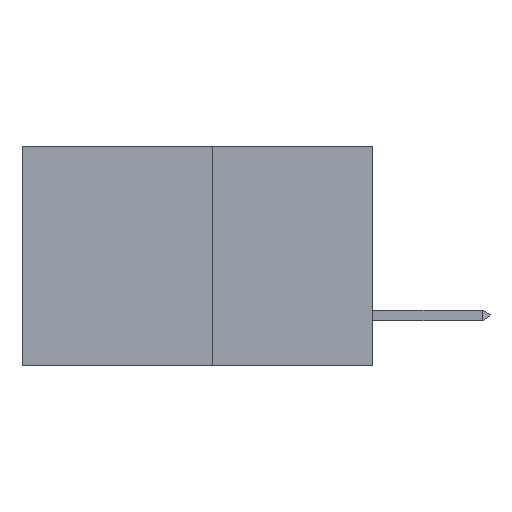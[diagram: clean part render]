
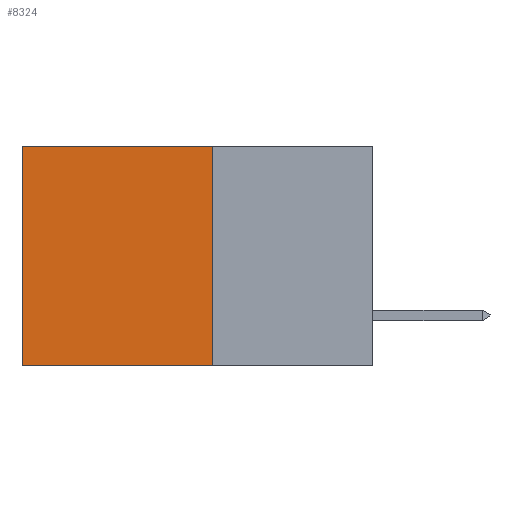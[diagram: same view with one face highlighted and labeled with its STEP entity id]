
A CAD part, left-side view. The second image highlights one B-rep face of the part: STEP entity #8324.
In plain terms, the highlighted planar face has unit normal (-1, 0, 0).
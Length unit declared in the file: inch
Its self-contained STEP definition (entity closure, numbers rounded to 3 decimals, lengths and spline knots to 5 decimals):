
#321 = VECTOR ( 'NONE', #8732, 39.37008 ) ;
#1023 = EDGE_CURVE ( 'NONE', #16219, #23307, #23272, .T. ) ;
#2029 = ORIENTED_EDGE ( 'NONE', *, *, #27375, .T. ) ;
#3308 = CARTESIAN_POINT ( 'NONE',  ( 0.277, 0.27, 0. ) ) ;
#4732 = LINE ( 'NONE', #7775, #20973 ) ;
#4986 = PLANE ( 'NONE',  #8059 ) ;
#6229 = EDGE_CURVE ( 'NONE', #21090, #7030, #11369, .T. ) ;
#7030 = VERTEX_POINT ( 'NONE', #16469 ) ;
#7775 = CARTESIAN_POINT ( 'NONE',  ( 0.277, 0.27, 0. ) ) ;
#8059 = AXIS2_PLACEMENT_3D ( 'NONE', #22584, #9438, #24719 ) ;
#8324 = ADVANCED_FACE ( 'NONE', ( #8785 ), #4986, .F. ) ;
#8732 = DIRECTION ( 'NONE',  ( 0., 0., -1. ) ) ;
#8767 = CARTESIAN_POINT ( 'NONE',  ( 0.277, 0.27, -0.37 ) ) ;
#8777 = ORIENTED_EDGE ( 'NONE', *, *, #9571, .F. ) ;
#8785 = FACE_OUTER_BOUND ( 'NONE', #26410, .T. ) ;
#9438 = DIRECTION ( 'NONE',  ( 1., 0., 0. ) ) ;
#9571 = EDGE_CURVE ( 'NONE', #7030, #23307, #25844, .T. ) ;
#9575 = DIRECTION ( 'NONE',  ( 0., 1., 0. ) ) ;
#11369 = LINE ( 'NONE', #8767, #321 ) ;
#13594 = ORIENTED_EDGE ( 'NONE', *, *, #6229, .F. ) ;
#14039 = DIRECTION ( 'NONE',  ( 0., 0., -1. ) ) ;
#14264 = CARTESIAN_POINT ( 'NONE',  ( 0.277, 0.59, -0.37 ) ) ;
#14354 = VECTOR ( 'NONE', #9575, 39.37008 ) ;
#15816 = CARTESIAN_POINT ( 'NONE',  ( 0.277, 0.59, -0.37 ) ) ;
#16219 = VERTEX_POINT ( 'NONE', #21399 ) ;
#16469 = CARTESIAN_POINT ( 'NONE',  ( 0.277, 0.27, -0.37 ) ) ;
#20973 = VECTOR ( 'NONE', #20998, 39.37008 ) ;
#20998 = DIRECTION ( 'NONE',  ( 0., 1., 0. ) ) ;
#21090 = VERTEX_POINT ( 'NONE', #3308 ) ;
#21399 = CARTESIAN_POINT ( 'NONE',  ( 0.277, 0.59, 0. ) ) ;
#22584 = CARTESIAN_POINT ( 'NONE',  ( 0.277, 0.27, -0.37 ) ) ;
#22601 = VECTOR ( 'NONE', #14039, 39.37008 ) ;
#23272 = LINE ( 'NONE', #14264, #22601 ) ;
#23307 = VERTEX_POINT ( 'NONE', #15816 ) ;
#24719 = DIRECTION ( 'NONE',  ( 0., 0., -1. ) ) ;
#24838 = CARTESIAN_POINT ( 'NONE',  ( 0.277, 0.27, -0.37 ) ) ;
#25844 = LINE ( 'NONE', #24838, #14354 ) ;
#26232 = ORIENTED_EDGE ( 'NONE', *, *, #1023, .T. ) ;
#26410 = EDGE_LOOP ( 'NONE', ( #26232, #8777, #13594, #2029 ) ) ;
#27375 = EDGE_CURVE ( 'NONE', #21090, #16219, #4732, .T. ) ;
